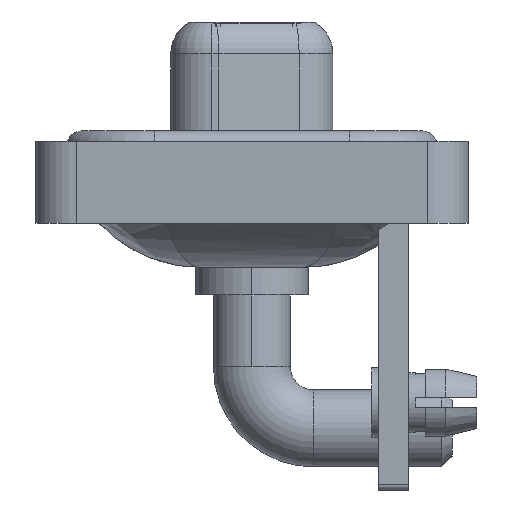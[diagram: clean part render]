
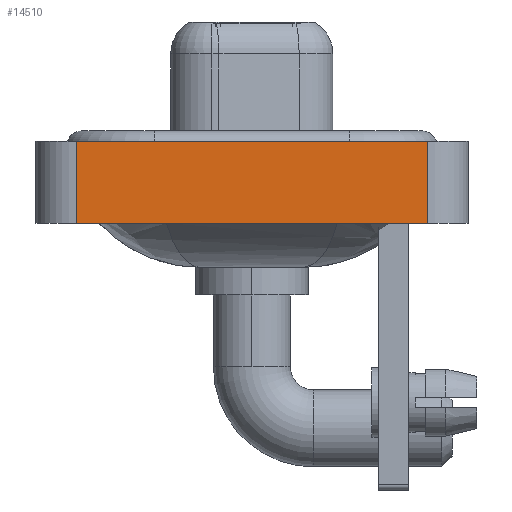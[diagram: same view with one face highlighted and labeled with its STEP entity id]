
A CAD part, left-side view. The second image highlights one B-rep face of the part: STEP entity #14510.
In plain terms, the highlighted planar face has unit normal (-1, 0, 0).
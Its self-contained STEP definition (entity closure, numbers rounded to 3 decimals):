
#474 = DIRECTION ( 'NONE',  ( 0., -1., 0. ) ) ;
#1905 = LINE ( 'NONE', #12370, #17759 ) ;
#2032 = LINE ( 'NONE', #13735, #9982 ) ;
#2283 = LINE ( 'NONE', #15533, #4000 ) ;
#2433 = VERTEX_POINT ( 'NONE', #4155 ) ;
#2739 = ORIENTED_EDGE ( 'NONE', *, *, #6918, .T. ) ;
#3406 = EDGE_LOOP ( 'NONE', ( #14744, #10563, #11801, #2739 ) ) ;
#4000 = VECTOR ( 'NONE', #8226, 1000. ) ;
#4155 = CARTESIAN_POINT ( 'NONE',  ( -7.35, -8.55, 0.4 ) ) ;
#4765 = FACE_OUTER_BOUND ( 'NONE', #3406, .T. ) ;
#6069 = VERTEX_POINT ( 'NONE', #16910 ) ;
#6918 = EDGE_CURVE ( 'NONE', #9236, #6069, #12161, .T. ) ;
#7840 = EDGE_CURVE ( 'NONE', #13001, #2433, #1905, .T. ) ;
#8226 = DIRECTION ( 'NONE',  ( 0., 0., 1. ) ) ;
#9236 = VERTEX_POINT ( 'NONE', #13497 ) ;
#9982 = VECTOR ( 'NONE', #12500, 1000. ) ;
#10563 = ORIENTED_EDGE ( 'NONE', *, *, #7840, .F. ) ;
#11801 = ORIENTED_EDGE ( 'NONE', *, *, #12197, .F. ) ;
#12161 = LINE ( 'NONE', #16469, #12214 ) ;
#12197 = EDGE_CURVE ( 'NONE', #9236, #13001, #2032, .T. ) ;
#12214 = VECTOR ( 'NONE', #18017, 1000. ) ;
#12256 = DIRECTION ( 'NONE',  ( -1., 0., 0. ) ) ;
#12370 = CARTESIAN_POINT ( 'NONE',  ( -7.35, -8.55, 0.4 ) ) ;
#12500 = DIRECTION ( 'NONE',  ( 0., 0., 1. ) ) ;
#13001 = VERTEX_POINT ( 'NONE', #17367 ) ;
#13204 = EDGE_CURVE ( 'NONE', #6069, #2433, #2283, .T. ) ;
#13497 = CARTESIAN_POINT ( 'NONE',  ( -7.35, 8.55, -3.6 ) ) ;
#13505 = DIRECTION ( 'NONE',  ( 0., 0., 1. ) ) ;
#13735 = CARTESIAN_POINT ( 'NONE',  ( -7.35, 8.55, -3.6 ) ) ;
#13891 = CARTESIAN_POINT ( 'NONE',  ( -7.35, -8.55, -3.6 ) ) ;
#14228 = AXIS2_PLACEMENT_3D ( 'NONE', #13891, #12256, #13505 ) ;
#14510 = ADVANCED_FACE ( 'NONE', ( #4765 ), #15335, .T. ) ;
#14744 = ORIENTED_EDGE ( 'NONE', *, *, #13204, .T. ) ;
#15335 = PLANE ( 'NONE',  #14228 ) ;
#15533 = CARTESIAN_POINT ( 'NONE',  ( -7.35, -8.55, -3.6 ) ) ;
#16469 = CARTESIAN_POINT ( 'NONE',  ( -7.35, -8.55, -3.6 ) ) ;
#16910 = CARTESIAN_POINT ( 'NONE',  ( -7.35, -8.55, -3.6 ) ) ;
#17367 = CARTESIAN_POINT ( 'NONE',  ( -7.35, 8.55, 0.4 ) ) ;
#17759 = VECTOR ( 'NONE', #474, 1000. ) ;
#18017 = DIRECTION ( 'NONE',  ( 0., -1., 0. ) ) ;
